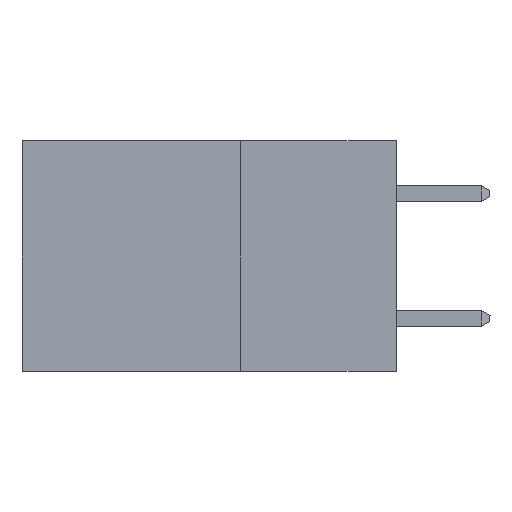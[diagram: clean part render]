
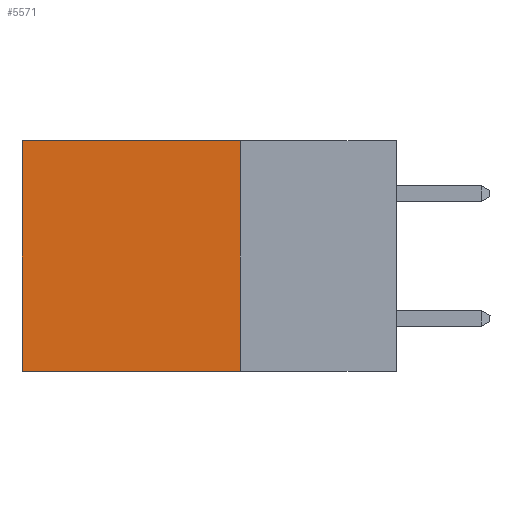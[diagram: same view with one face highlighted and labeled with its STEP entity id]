
A CAD part, left-side view. The second image highlights one B-rep face of the part: STEP entity #5571.
In plain terms, the highlighted planar face has unit normal (-1, 0, 0).
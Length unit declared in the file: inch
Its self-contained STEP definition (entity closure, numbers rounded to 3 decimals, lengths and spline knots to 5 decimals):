
#84 = EDGE_CURVE ( 'NONE', #7311, #7847, #8235, .T. ) ;
#200 = CARTESIAN_POINT ( 'NONE',  ( 0.2615, 0.6, -0.37 ) ) ;
#388 = CARTESIAN_POINT ( 'NONE',  ( 0.2615, 0.25, -0.37 ) ) ;
#1604 = DIRECTION ( 'NONE',  ( 0., 1., 0. ) ) ;
#1957 = ORIENTED_EDGE ( 'NONE', *, *, #7373, .T. ) ;
#2681 = FACE_OUTER_BOUND ( 'NONE', #6390, .T. ) ;
#3172 = PLANE ( 'NONE',  #10221 ) ;
#3721 = ORIENTED_EDGE ( 'NONE', *, *, #10556, .F. ) ;
#4073 = VECTOR ( 'NONE', #9439, 39.37008 ) ;
#4293 = VECTOR ( 'NONE', #1604, 39.37008 ) ;
#4296 = CARTESIAN_POINT ( 'NONE',  ( 0.2615, 0.25, -0.37 ) ) ;
#4598 = CARTESIAN_POINT ( 'NONE',  ( 0.2615, 0.6, -0.37 ) ) ;
#4614 = VECTOR ( 'NONE', #10389, 39.37008 ) ;
#4643 = CARTESIAN_POINT ( 'NONE',  ( 0.2615, 0.25, 0. ) ) ;
#4864 = DIRECTION ( 'NONE',  ( 0., 0., -1. ) ) ;
#4958 = VERTEX_POINT ( 'NONE', #7859 ) ;
#5571 = ADVANCED_FACE ( 'NONE', ( #2681 ), #3172, .F. ) ;
#5720 = ORIENTED_EDGE ( 'NONE', *, *, #8015, .F. ) ;
#6168 = VECTOR ( 'NONE', #8766, 39.37008 ) ;
#6390 = EDGE_LOOP ( 'NONE', ( #9087, #3721, #5720, #1957 ) ) ;
#6515 = VERTEX_POINT ( 'NONE', #4296 ) ;
#6535 = LINE ( 'NONE', #8281, #4293 ) ;
#7311 = VERTEX_POINT ( 'NONE', #8566 ) ;
#7373 = EDGE_CURVE ( 'NONE', #4958, #7311, #10645, .T. ) ;
#7847 = VERTEX_POINT ( 'NONE', #200 ) ;
#7859 = CARTESIAN_POINT ( 'NONE',  ( 0.2615, 0.25, 0. ) ) ;
#8015 = EDGE_CURVE ( 'NONE', #4958, #6515, #10506, .T. ) ;
#8235 = LINE ( 'NONE', #4598, #4073 ) ;
#8281 = CARTESIAN_POINT ( 'NONE',  ( 0.2615, 0.25, -0.37 ) ) ;
#8566 = CARTESIAN_POINT ( 'NONE',  ( 0.2615, 0.6, 0. ) ) ;
#8766 = DIRECTION ( 'NONE',  ( 0., 0., -1. ) ) ;
#8998 = CARTESIAN_POINT ( 'NONE',  ( 0.2615, 0.25, -0.37 ) ) ;
#9087 = ORIENTED_EDGE ( 'NONE', *, *, #84, .T. ) ;
#9439 = DIRECTION ( 'NONE',  ( 0., 0., -1. ) ) ;
#9792 = DIRECTION ( 'NONE',  ( 1., 0., 0. ) ) ;
#10221 = AXIS2_PLACEMENT_3D ( 'NONE', #8998, #9792, #4864 ) ;
#10389 = DIRECTION ( 'NONE',  ( 0., 1., 0. ) ) ;
#10506 = LINE ( 'NONE', #388, #6168 ) ;
#10556 = EDGE_CURVE ( 'NONE', #6515, #7847, #6535, .T. ) ;
#10645 = LINE ( 'NONE', #4643, #4614 ) ;
